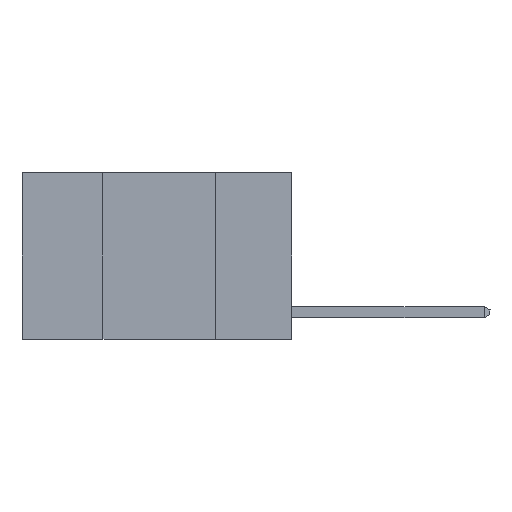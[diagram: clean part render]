
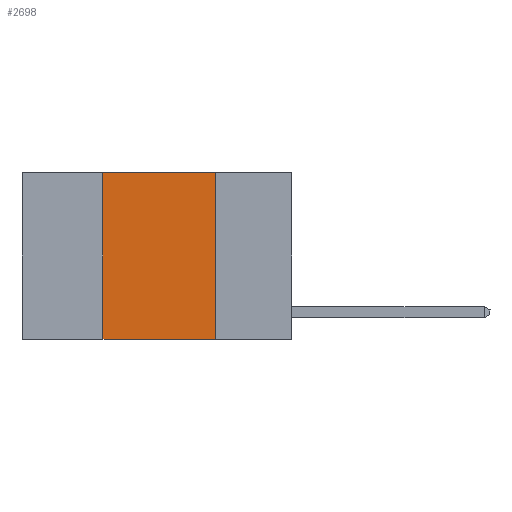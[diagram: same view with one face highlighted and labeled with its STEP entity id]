
A CAD part, left-side view. The second image highlights one B-rep face of the part: STEP entity #2698.
In plain terms, the highlighted planar face has unit normal (-1, 0, 0).
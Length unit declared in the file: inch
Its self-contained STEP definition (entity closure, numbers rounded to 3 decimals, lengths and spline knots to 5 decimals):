
#809 = FACE_OUTER_BOUND ( 'NONE', #17668, .T. ) ;
#822 = PLANE ( 'NONE',  #25417 ) ;
#1084 = CARTESIAN_POINT ( 'NONE',  ( 0., 0.6, 0. ) ) ;
#2163 = EDGE_CURVE ( 'NONE', #21796, #19561, #7811, .T. ) ;
#2698 = ADVANCED_FACE ( 'NONE', ( #809 ), #822, .F. ) ;
#2871 = EDGE_CURVE ( 'NONE', #7087, #11642, #10017, .T. ) ;
#3343 = DIRECTION ( 'NONE',  ( 0., 0., -1. ) ) ;
#3349 = VECTOR ( 'NONE', #24746, 39.37008 ) ;
#3872 = DIRECTION ( 'NONE',  ( 0., 0., 1. ) ) ;
#4904 = VECTOR ( 'NONE', #3872, 39.37008 ) ;
#5037 = ORIENTED_EDGE ( 'NONE', *, *, #20005, .T. ) ;
#5899 = ORIENTED_EDGE ( 'NONE', *, *, #19652, .F. ) ;
#7087 = VERTEX_POINT ( 'NONE', #19936 ) ;
#7811 = LINE ( 'NONE', #13252, #13881 ) ;
#9035 = CARTESIAN_POINT ( 'NONE',  ( 0., 0.42, 0. ) ) ;
#9292 = DIRECTION ( 'NONE',  ( 0., 0., -1. ) ) ;
#9427 = CARTESIAN_POINT ( 'NONE',  ( 0., 0.17, 0. ) ) ;
#10017 = LINE ( 'NONE', #24750, #4904 ) ;
#10374 = CARTESIAN_POINT ( 'NONE',  ( 0., 0.6, -0.37 ) ) ;
#11642 = VERTEX_POINT ( 'NONE', #9035 ) ;
#11741 = ORIENTED_EDGE ( 'NONE', *, *, #2871, .F. ) ;
#12561 = CARTESIAN_POINT ( 'NONE',  ( 0., 0.6, 0. ) ) ;
#13252 = CARTESIAN_POINT ( 'NONE',  ( 0., 0.17, 0. ) ) ;
#13256 = LINE ( 'NONE', #12561, #19337 ) ;
#13881 = VECTOR ( 'NONE', #3343, 39.37008 ) ;
#14811 = LINE ( 'NONE', #10374, #3349 ) ;
#16588 = DIRECTION ( 'NONE',  ( 0., -1., 0. ) ) ;
#17253 = DIRECTION ( 'NONE',  ( 1., 0., 0. ) ) ;
#17668 = EDGE_LOOP ( 'NONE', ( #22408, #5899, #11741, #5037 ) ) ;
#19337 = VECTOR ( 'NONE', #16588, 39.37008 ) ;
#19561 = VERTEX_POINT ( 'NONE', #24817 ) ;
#19652 = EDGE_CURVE ( 'NONE', #11642, #21796, #13256, .T. ) ;
#19936 = CARTESIAN_POINT ( 'NONE',  ( 0., 0.42, -0.37 ) ) ;
#20005 = EDGE_CURVE ( 'NONE', #7087, #19561, #14811, .T. ) ;
#21796 = VERTEX_POINT ( 'NONE', #9427 ) ;
#22408 = ORIENTED_EDGE ( 'NONE', *, *, #2163, .F. ) ;
#24746 = DIRECTION ( 'NONE',  ( 0., -1., 0. ) ) ;
#24750 = CARTESIAN_POINT ( 'NONE',  ( 0., 0.42, 0. ) ) ;
#24817 = CARTESIAN_POINT ( 'NONE',  ( 0., 0.17, -0.37 ) ) ;
#25417 = AXIS2_PLACEMENT_3D ( 'NONE', #1084, #17253, #9292 ) ;
